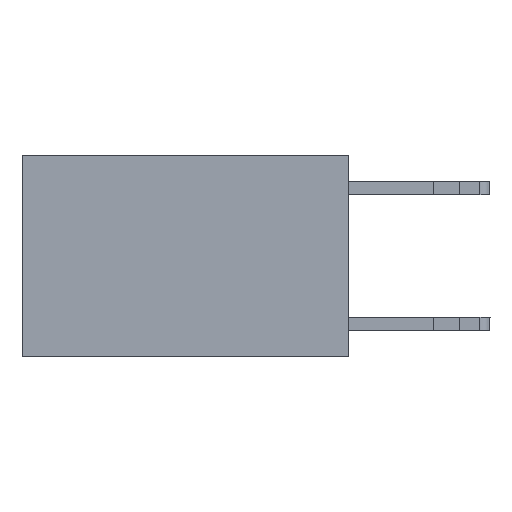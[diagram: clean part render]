
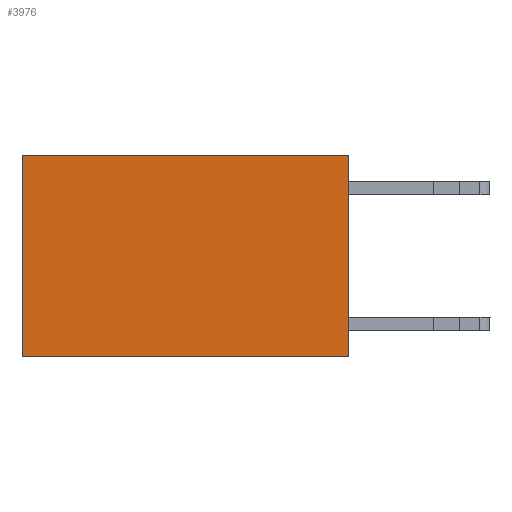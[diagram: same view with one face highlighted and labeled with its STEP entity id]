
A CAD part, left-side view. The second image highlights one B-rep face of the part: STEP entity #3976.
In plain terms, the highlighted planar face has unit normal (-1, 0, 0).
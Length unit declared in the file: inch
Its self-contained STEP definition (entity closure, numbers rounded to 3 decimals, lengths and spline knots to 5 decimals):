
#765 = PLANE ( 'NONE',  #21249 ) ;
#1832 = CARTESIAN_POINT ( 'NONE',  ( 0.2625, 0.6, 0. ) ) ;
#2224 = FACE_OUTER_BOUND ( 'NONE', #20989, .T. ) ;
#3064 = VERTEX_POINT ( 'NONE', #15185 ) ;
#3145 = CARTESIAN_POINT ( 'NONE',  ( 0.2625, 0., 0. ) ) ;
#3976 = ADVANCED_FACE ( 'NONE', ( #2224 ), #765, .F. ) ;
#4314 = ORIENTED_EDGE ( 'NONE', *, *, #22579, .T. ) ;
#4379 = VECTOR ( 'NONE', #5084, 39.37008 ) ;
#4554 = DIRECTION ( 'NONE',  ( 0., 0., -1. ) ) ;
#5084 = DIRECTION ( 'NONE',  ( 0., 1., 0. ) ) ;
#7141 = CARTESIAN_POINT ( 'NONE',  ( 0.2625, 0., 0. ) ) ;
#7903 = CARTESIAN_POINT ( 'NONE',  ( 0.2625, 0.6, -0.37 ) ) ;
#8315 = LINE ( 'NONE', #3145, #4379 ) ;
#9100 = DIRECTION ( 'NONE',  ( 0., 0., -1. ) ) ;
#10545 = DIRECTION ( 'NONE',  ( 1., 0., 0. ) ) ;
#12248 = VERTEX_POINT ( 'NONE', #7903 ) ;
#12356 = LINE ( 'NONE', #14266, #22001 ) ;
#12478 = VECTOR ( 'NONE', #14768, 39.37008 ) ;
#12773 = CARTESIAN_POINT ( 'NONE',  ( 0.2625, 0., -0.37 ) ) ;
#13350 = VECTOR ( 'NONE', #9100, 39.37008 ) ;
#13984 = LINE ( 'NONE', #7141, #13350 ) ;
#14266 = CARTESIAN_POINT ( 'NONE',  ( 0.2625, 0.6, 0. ) ) ;
#14768 = DIRECTION ( 'NONE',  ( 0., 1., 0. ) ) ;
#15185 = CARTESIAN_POINT ( 'NONE',  ( 0.2625, 0., 0. ) ) ;
#16100 = EDGE_CURVE ( 'NONE', #22235, #12248, #18240, .T. ) ;
#16715 = EDGE_CURVE ( 'NONE', #3064, #22235, #13984, .T. ) ;
#18240 = LINE ( 'NONE', #12773, #12478 ) ;
#18310 = ORIENTED_EDGE ( 'NONE', *, *, #16100, .F. ) ;
#18374 = EDGE_CURVE ( 'NONE', #23386, #12248, #12356, .T. ) ;
#20157 = CARTESIAN_POINT ( 'NONE',  ( 0.2625, 0., 0. ) ) ;
#20989 = EDGE_LOOP ( 'NONE', ( #23531, #18310, #23314, #4314 ) ) ;
#21249 = AXIS2_PLACEMENT_3D ( 'NONE', #20157, #10545, #23997 ) ;
#22001 = VECTOR ( 'NONE', #4554, 39.37008 ) ;
#22235 = VERTEX_POINT ( 'NONE', #23796 ) ;
#22579 = EDGE_CURVE ( 'NONE', #3064, #23386, #8315, .T. ) ;
#23314 = ORIENTED_EDGE ( 'NONE', *, *, #16715, .F. ) ;
#23386 = VERTEX_POINT ( 'NONE', #1832 ) ;
#23531 = ORIENTED_EDGE ( 'NONE', *, *, #18374, .T. ) ;
#23796 = CARTESIAN_POINT ( 'NONE',  ( 0.2625, 0., -0.37 ) ) ;
#23997 = DIRECTION ( 'NONE',  ( 0., 0., -1. ) ) ;
